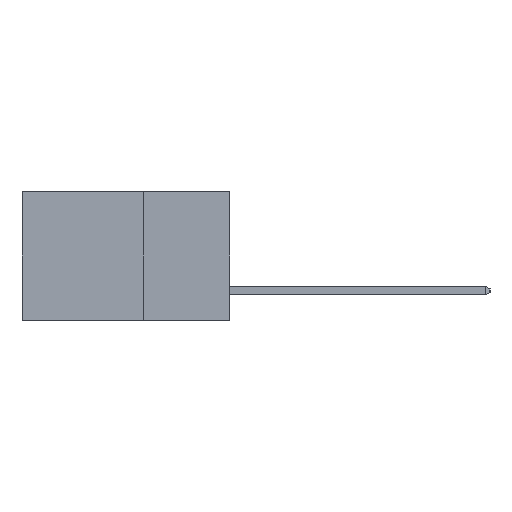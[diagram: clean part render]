
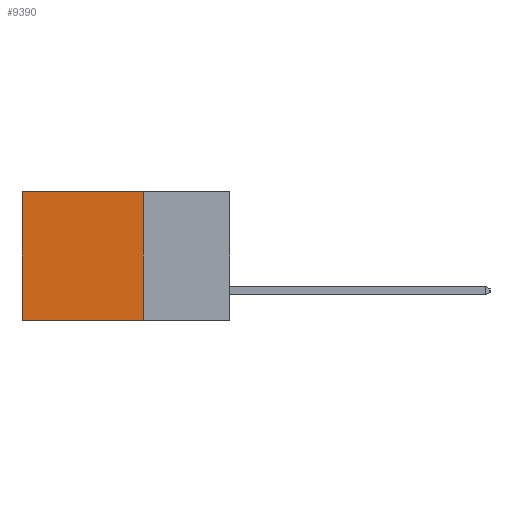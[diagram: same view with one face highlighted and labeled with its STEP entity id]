
A CAD part, left-side view. The second image highlights one B-rep face of the part: STEP entity #9390.
In plain terms, the highlighted planar face has unit normal (-1, 0, 0).
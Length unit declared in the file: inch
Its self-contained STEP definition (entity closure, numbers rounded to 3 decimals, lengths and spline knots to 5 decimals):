
#604 = EDGE_CURVE ( 'NONE', #13847, #9105, #11100, .T. ) ;
#657 = LINE ( 'NONE', #11004, #7118 ) ;
#1334 = VERTEX_POINT ( 'NONE', #15098 ) ;
#1532 = VERTEX_POINT ( 'NONE', #8048 ) ;
#1538 = ORIENTED_EDGE ( 'NONE', *, *, #7122, .T. ) ;
#1775 = EDGE_CURVE ( 'NONE', #13847, #1532, #657, .T. ) ;
#1846 = ORIENTED_EDGE ( 'NONE', *, *, #14645, .F. ) ;
#2261 = ORIENTED_EDGE ( 'NONE', *, *, #1775, .F. ) ;
#2441 = CARTESIAN_POINT ( 'NONE',  ( 0.298, 0.6, 0. ) ) ;
#2549 = DIRECTION ( 'NONE',  ( 0., 0., -1. ) ) ;
#2692 = ORIENTED_EDGE ( 'NONE', *, *, #604, .T. ) ;
#4460 = LINE ( 'NONE', #13932, #7332 ) ;
#7118 = VECTOR ( 'NONE', #11847, 39.37008 ) ;
#7122 = EDGE_CURVE ( 'NONE', #9105, #1334, #11166, .T. ) ;
#7277 = FACE_OUTER_BOUND ( 'NONE', #13731, .T. ) ;
#7300 = AXIS2_PLACEMENT_3D ( 'NONE', #10931, #10682, #10671 ) ;
#7332 = VECTOR ( 'NONE', #13981, 39.37008 ) ;
#8048 = CARTESIAN_POINT ( 'NONE',  ( 0.298, 0.25, -0.37 ) ) ;
#8084 = VECTOR ( 'NONE', #10297, 39.37008 ) ;
#8532 = VECTOR ( 'NONE', #2549, 39.37008 ) ;
#9021 = CARTESIAN_POINT ( 'NONE',  ( 0.298, 0.25, 0. ) ) ;
#9105 = VERTEX_POINT ( 'NONE', #14660 ) ;
#9185 = CARTESIAN_POINT ( 'NONE',  ( 0.298, 0.25, 0. ) ) ;
#9390 = ADVANCED_FACE ( 'NONE', ( #7277 ), #10717, .F. ) ;
#10297 = DIRECTION ( 'NONE',  ( 0., 1., 0. ) ) ;
#10671 = DIRECTION ( 'NONE',  ( 0., 0., -1. ) ) ;
#10682 = DIRECTION ( 'NONE',  ( 1., 0., 0. ) ) ;
#10717 = PLANE ( 'NONE',  #7300 ) ;
#10931 = CARTESIAN_POINT ( 'NONE',  ( 0.298, 0.25, 0. ) ) ;
#11004 = CARTESIAN_POINT ( 'NONE',  ( 0.298, 0.25, 0. ) ) ;
#11100 = LINE ( 'NONE', #9185, #8084 ) ;
#11166 = LINE ( 'NONE', #2441, #8532 ) ;
#11847 = DIRECTION ( 'NONE',  ( 0., 0., -1. ) ) ;
#13731 = EDGE_LOOP ( 'NONE', ( #1538, #1846, #2261, #2692 ) ) ;
#13847 = VERTEX_POINT ( 'NONE', #9021 ) ;
#13932 = CARTESIAN_POINT ( 'NONE',  ( 0.298, 0.25, -0.37 ) ) ;
#13981 = DIRECTION ( 'NONE',  ( 0., 1., 0. ) ) ;
#14645 = EDGE_CURVE ( 'NONE', #1532, #1334, #4460, .T. ) ;
#14660 = CARTESIAN_POINT ( 'NONE',  ( 0.298, 0.6, 0. ) ) ;
#15098 = CARTESIAN_POINT ( 'NONE',  ( 0.298, 0.6, -0.37 ) ) ;
